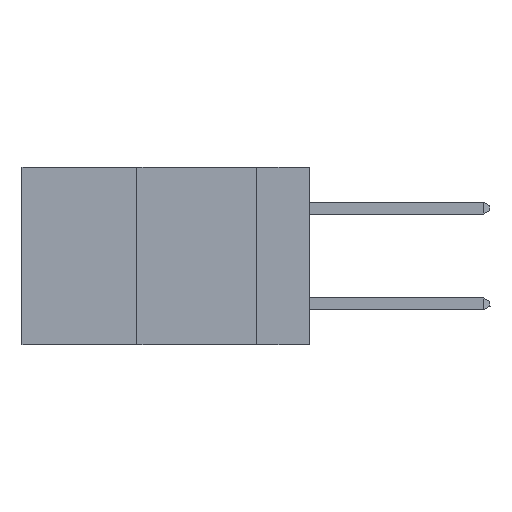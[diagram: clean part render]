
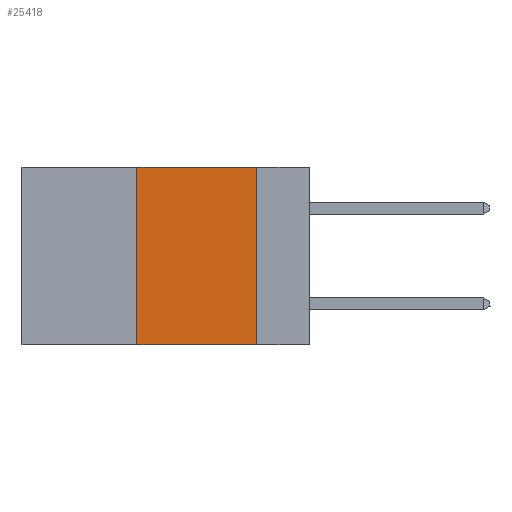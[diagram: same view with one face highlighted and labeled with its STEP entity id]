
A CAD part, left-side view. The second image highlights one B-rep face of the part: STEP entity #25418.
In plain terms, the highlighted planar face has unit normal (-1, 0, 0).
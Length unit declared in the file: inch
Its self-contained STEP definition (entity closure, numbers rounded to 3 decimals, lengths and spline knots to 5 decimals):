
#5 = EDGE_CURVE ( 'NONE', #18778, #21530, #27315, .T. ) ;
#44 = LINE ( 'NONE', #12516, #11406 ) ;
#785 = VECTOR ( 'NONE', #3058, 39.37008 ) ;
#977 = PLANE ( 'NONE',  #13269 ) ;
#2792 = DIRECTION ( 'NONE',  ( 0., -1., 0. ) ) ;
#2801 = ORIENTED_EDGE ( 'NONE', *, *, #28595, .F. ) ;
#3058 = DIRECTION ( 'NONE',  ( 0., -1., 0. ) ) ;
#3557 = VERTEX_POINT ( 'NONE', #8827 ) ;
#4452 = CARTESIAN_POINT ( 'NONE',  ( 0., 0.36, 0. ) ) ;
#6958 = ORIENTED_EDGE ( 'NONE', *, *, #29212, .F. ) ;
#8827 = CARTESIAN_POINT ( 'NONE',  ( 0., 0.11, 0. ) ) ;
#8925 = DIRECTION ( 'NONE',  ( 0., 0., -1. ) ) ;
#9524 = EDGE_LOOP ( 'NONE', ( #6958, #2801, #26972, #30848 ) ) ;
#9558 = VERTEX_POINT ( 'NONE', #26937 ) ;
#9821 = VECTOR ( 'NONE', #2792, 39.37008 ) ;
#11323 = DIRECTION ( 'NONE',  ( 1., 0., 0. ) ) ;
#11406 = VECTOR ( 'NONE', #30774, 39.37008 ) ;
#11439 = CARTESIAN_POINT ( 'NONE',  ( 0., 0.6, 0. ) ) ;
#12516 = CARTESIAN_POINT ( 'NONE',  ( 0., 0.11, 0. ) ) ;
#13269 = AXIS2_PLACEMENT_3D ( 'NONE', #11439, #11323, #8925 ) ;
#13373 = CARTESIAN_POINT ( 'NONE',  ( 0., 0.6, -0.37 ) ) ;
#13529 = CARTESIAN_POINT ( 'NONE',  ( 0., 0.11, -0.37 ) ) ;
#18369 = CARTESIAN_POINT ( 'NONE',  ( 0., 0.6, 0. ) ) ;
#18778 = VERTEX_POINT ( 'NONE', #33370 ) ;
#19381 = FACE_OUTER_BOUND ( 'NONE', #9524, .T. ) ;
#21530 = VERTEX_POINT ( 'NONE', #13529 ) ;
#22701 = LINE ( 'NONE', #4452, #28020 ) ;
#22874 = DIRECTION ( 'NONE',  ( 0., 0., 1. ) ) ;
#25418 = ADVANCED_FACE ( 'NONE', ( #19381 ), #977, .F. ) ;
#26937 = CARTESIAN_POINT ( 'NONE',  ( 0., 0.36, 0. ) ) ;
#26972 = ORIENTED_EDGE ( 'NONE', *, *, #32981, .F. ) ;
#27315 = LINE ( 'NONE', #13373, #785 ) ;
#28020 = VECTOR ( 'NONE', #22874, 39.37008 ) ;
#28195 = LINE ( 'NONE', #18369, #9821 ) ;
#28595 = EDGE_CURVE ( 'NONE', #9558, #3557, #28195, .T. ) ;
#29212 = EDGE_CURVE ( 'NONE', #3557, #21530, #44, .T. ) ;
#30774 = DIRECTION ( 'NONE',  ( 0., 0., -1. ) ) ;
#30848 = ORIENTED_EDGE ( 'NONE', *, *, #5, .T. ) ;
#32981 = EDGE_CURVE ( 'NONE', #18778, #9558, #22701, .T. ) ;
#33370 = CARTESIAN_POINT ( 'NONE',  ( 0., 0.36, -0.37 ) ) ;
